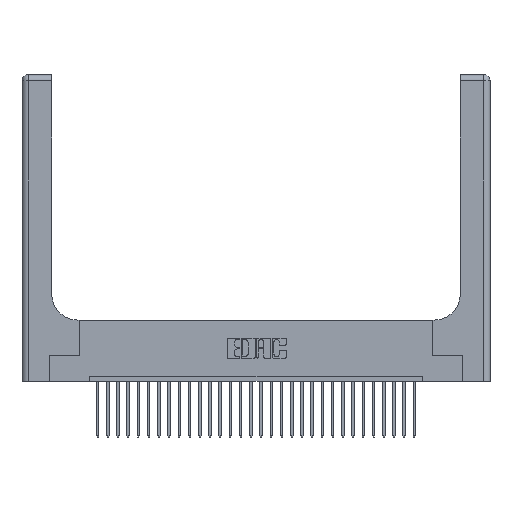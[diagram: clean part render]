
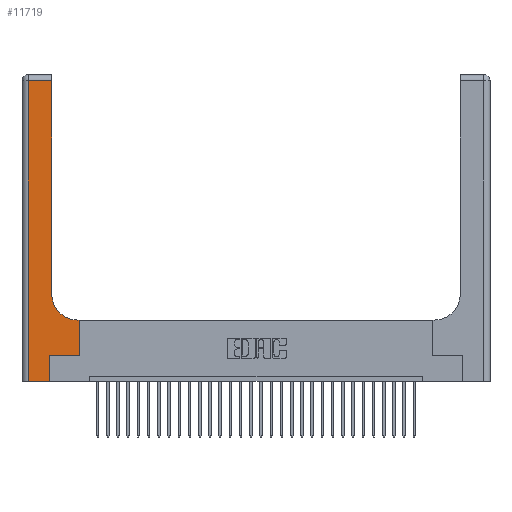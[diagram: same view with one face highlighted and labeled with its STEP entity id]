
A CAD part, top view. The second image highlights one B-rep face of the part: STEP entity #11719.
In plain terms, the highlighted planar face has unit normal (0, 0, 1).
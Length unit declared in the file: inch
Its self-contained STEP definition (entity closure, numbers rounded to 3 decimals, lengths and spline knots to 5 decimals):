
#343 = CARTESIAN_POINT ( 'NONE',  ( 0.06, 0., 0.37 ) ) ;
#531 = CARTESIAN_POINT ( 'NONE',  ( 0.5415, 0.6, 0.37 ) ) ;
#702 = EDGE_LOOP ( 'NONE', ( #938, #26136, #13743, #17830, #19597, #23113, #2075, #13517, #9388 ) ) ;
#835 = CARTESIAN_POINT ( 'NONE',  ( 0.2915, 0.85, 0.37 ) ) ;
#938 = ORIENTED_EDGE ( 'NONE', *, *, #14181, .T. ) ;
#1519 = CARTESIAN_POINT ( 'NONE',  ( 0.269, 0., 0.37 ) ) ;
#2075 = ORIENTED_EDGE ( 'NONE', *, *, #24093, .T. ) ;
#2494 = CARTESIAN_POINT ( 'NONE',  ( 0.5415, 0.85, 0.37 ) ) ;
#2594 = DIRECTION ( 'NONE',  ( 0., 0., -1. ) ) ;
#3304 = PLANE ( 'NONE',  #13724 ) ;
#4626 = VERTEX_POINT ( 'NONE', #21984 ) ;
#5392 = DIRECTION ( 'NONE',  ( -1., 0., 0. ) ) ;
#6260 = VECTOR ( 'NONE', #11294, 39.37008 ) ;
#6348 = DIRECTION ( 'NONE',  ( 0., 1., 0. ) ) ;
#6440 = VECTOR ( 'NONE', #5392, 39.37008 ) ;
#6836 = EDGE_CURVE ( 'NONE', #12197, #28315, #22892, .T. ) ;
#6995 = CARTESIAN_POINT ( 'NONE',  ( 0.06, 3., 0.37 ) ) ;
#7103 = FACE_OUTER_BOUND ( 'NONE', #702, .T. ) ;
#7467 = VERTEX_POINT ( 'NONE', #343 ) ;
#8713 = CARTESIAN_POINT ( 'NONE',  ( 0.269, 0.25, 0.37 ) ) ;
#9267 = CARTESIAN_POINT ( 'NONE',  ( 0.269, 0.25, 0.37 ) ) ;
#9349 = VECTOR ( 'NONE', #30365, 39.37008 ) ;
#9388 = ORIENTED_EDGE ( 'NONE', *, *, #9911, .T. ) ;
#9911 = EDGE_CURVE ( 'NONE', #27815, #13819, #10532, .T. ) ;
#10149 = VECTOR ( 'NONE', #11441, 39.37008 ) ;
#10416 = EDGE_CURVE ( 'NONE', #21750, #27815, #17121, .T. ) ;
#10479 = CARTESIAN_POINT ( 'NONE',  ( 0.5585, 0.25, 0.37 ) ) ;
#10532 = CIRCLE ( 'NONE', #30525, 0.25 ) ;
#10709 = VECTOR ( 'NONE', #6348, 39.37008 ) ;
#10885 = CARTESIAN_POINT ( 'NONE',  ( 0.5585, 0.25, 0.37 ) ) ;
#11294 = DIRECTION ( 'NONE',  ( 1., 0., 0. ) ) ;
#11441 = DIRECTION ( 'NONE',  ( 0., -1., 0. ) ) ;
#11446 = LINE ( 'NONE', #10885, #10709 ) ;
#11719 = ADVANCED_FACE ( 'NONE', ( #7103 ), #3304, .F. ) ;
#12144 = CARTESIAN_POINT ( 'NONE',  ( 0.2915, 3., 0.37 ) ) ;
#12197 = VERTEX_POINT ( 'NONE', #9267 ) ;
#12784 = DIRECTION ( 'NONE',  ( 0., 0., -1. ) ) ;
#13186 = DIRECTION ( 'NONE',  ( 0., 1., 0. ) ) ;
#13419 = VERTEX_POINT ( 'NONE', #28913 ) ;
#13517 = ORIENTED_EDGE ( 'NONE', *, *, #10416, .T. ) ;
#13724 = AXIS2_PLACEMENT_3D ( 'NONE', #29007, #12784, #14957 ) ;
#13733 = LINE ( 'NONE', #25447, #9349 ) ;
#13743 = ORIENTED_EDGE ( 'NONE', *, *, #30617, .T. ) ;
#13819 = VERTEX_POINT ( 'NONE', #835 ) ;
#14181 = EDGE_CURVE ( 'NONE', #13819, #13419, #29830, .T. ) ;
#14783 = LINE ( 'NONE', #1519, #24425 ) ;
#14957 = DIRECTION ( 'NONE',  ( -1., 0., 0. ) ) ;
#17116 = EDGE_CURVE ( 'NONE', #13419, #20049, #13733, .T. ) ;
#17121 = LINE ( 'NONE', #24399, #6440 ) ;
#17341 = CARTESIAN_POINT ( 'NONE',  ( 0., 0., 0.37 ) ) ;
#17830 = ORIENTED_EDGE ( 'NONE', *, *, #29794, .T. ) ;
#18371 = VECTOR ( 'NONE', #19220, 39.37008 ) ;
#18680 = CARTESIAN_POINT ( 'NONE',  ( 0.06, 2.94, 0.37 ) ) ;
#19220 = DIRECTION ( 'NONE',  ( 0., 1., 0. ) ) ;
#19597 = ORIENTED_EDGE ( 'NONE', *, *, #26235, .T. ) ;
#20049 = VERTEX_POINT ( 'NONE', #18680 ) ;
#20705 = DIRECTION ( 'NONE',  ( 1., 0., 0. ) ) ;
#21750 = VERTEX_POINT ( 'NONE', #24658 ) ;
#21984 = CARTESIAN_POINT ( 'NONE',  ( 0.269, 0., 0.37 ) ) ;
#22892 = LINE ( 'NONE', #8713, #6260 ) ;
#23113 = ORIENTED_EDGE ( 'NONE', *, *, #6836, .T. ) ;
#23543 = VECTOR ( 'NONE', #20705, 39.37008 ) ;
#24093 = EDGE_CURVE ( 'NONE', #28315, #21750, #11446, .T. ) ;
#24399 = CARTESIAN_POINT ( 'NONE',  ( 0.2915, 0.6, 0.37 ) ) ;
#24425 = VECTOR ( 'NONE', #13186, 39.37008 ) ;
#24658 = CARTESIAN_POINT ( 'NONE',  ( 0.5585, 0.6, 0.37 ) ) ;
#25312 = LINE ( 'NONE', #6995, #10149 ) ;
#25447 = CARTESIAN_POINT ( 'NONE',  ( 0., 2.94, 0.37 ) ) ;
#26136 = ORIENTED_EDGE ( 'NONE', *, *, #17116, .T. ) ;
#26149 = DIRECTION ( 'NONE',  ( 1., 0., 0. ) ) ;
#26235 = EDGE_CURVE ( 'NONE', #4626, #12197, #14783, .T. ) ;
#26818 = LINE ( 'NONE', #17341, #23543 ) ;
#27815 = VERTEX_POINT ( 'NONE', #531 ) ;
#28315 = VERTEX_POINT ( 'NONE', #10479 ) ;
#28913 = CARTESIAN_POINT ( 'NONE',  ( 0.2915, 2.94, 0.37 ) ) ;
#29007 = CARTESIAN_POINT ( 'NONE',  ( 0., 3., 0.37 ) ) ;
#29794 = EDGE_CURVE ( 'NONE', #7467, #4626, #26818, .T. ) ;
#29830 = LINE ( 'NONE', #12144, #18371 ) ;
#30365 = DIRECTION ( 'NONE',  ( -1., 0., 0. ) ) ;
#30525 = AXIS2_PLACEMENT_3D ( 'NONE', #2494, #2594, #26149 ) ;
#30617 = EDGE_CURVE ( 'NONE', #20049, #7467, #25312, .T. ) ;
